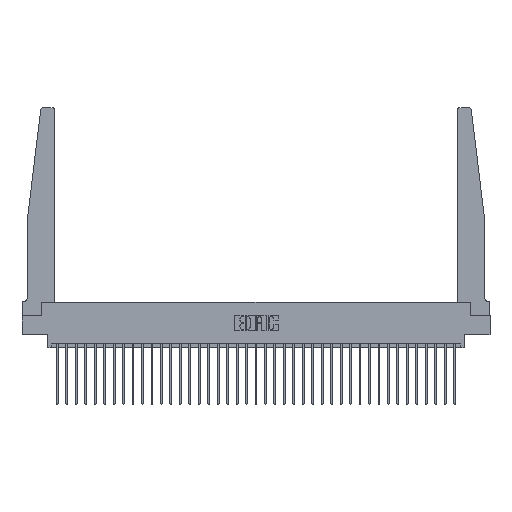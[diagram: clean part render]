
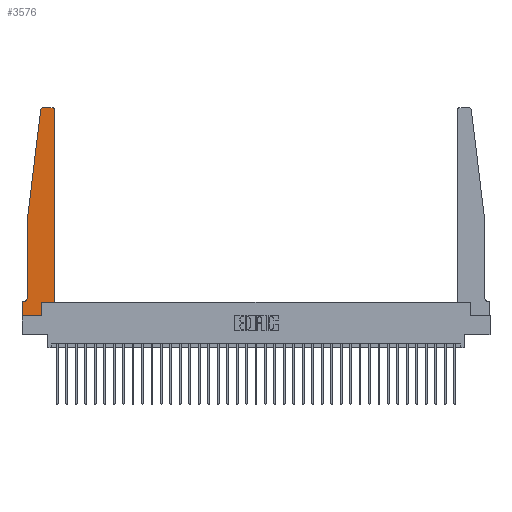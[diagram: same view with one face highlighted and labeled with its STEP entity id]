
A CAD part, top view. The second image highlights one B-rep face of the part: STEP entity #3576.
In plain terms, the highlighted planar face has unit normal (0, 0, 1).
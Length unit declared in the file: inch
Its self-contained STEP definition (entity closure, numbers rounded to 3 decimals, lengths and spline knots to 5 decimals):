
#4 = EDGE_CURVE ( 'NONE', #29340, #1644, #8275, .T. ) ;
#60 = CARTESIAN_POINT ( 'NONE',  ( 0.25, 2.75, 0.37 ) ) ;
#529 = VECTOR ( 'NONE', #12540, 39.37008 ) ;
#1047 = LINE ( 'NONE', #10996, #31137 ) ;
#1213 = EDGE_CURVE ( 'NONE', #19948, #30841, #32420, .T. ) ;
#1644 = VERTEX_POINT ( 'NONE', #14336 ) ;
#1823 = EDGE_CURVE ( 'NONE', #9716, #26521, #4570, .T. ) ;
#2283 = CARTESIAN_POINT ( 'NONE',  ( 0.425, 0.18, 0.37 ) ) ;
#2417 = EDGE_CURVE ( 'NONE', #14620, #32169, #27530, .T. ) ;
#2706 = LINE ( 'NONE', #31179, #25976 ) ;
#2826 = VERTEX_POINT ( 'NONE', #11321 ) ;
#3506 = CARTESIAN_POINT ( 'NONE',  ( 0.425, 0.18, 0.37 ) ) ;
#3576 = ADVANCED_FACE ( 'NONE', ( #8250 ), #26257, .T. ) ;
#3982 = CARTESIAN_POINT ( 'NONE',  ( 0., 0.1875, 0.37 ) ) ;
#4303 = CARTESIAN_POINT ( 'NONE',  ( 0.425, 0.18, 0.37 ) ) ;
#4419 = AXIS2_PLACEMENT_3D ( 'NONE', #22112, #9162, #19418 ) ;
#4570 = CIRCLE ( 'NONE', #27695, 0.03 ) ;
#5114 = VERTEX_POINT ( 'NONE', #31944 ) ;
#5246 = VECTOR ( 'NONE', #18828, 39.37008 ) ;
#5378 = CARTESIAN_POINT ( 'NONE',  ( 0.27653, 2.75, 0.37 ) ) ;
#5499 = VECTOR ( 'NONE', #24867, 39.37008 ) ;
#6516 = EDGE_CURVE ( 'NONE', #22549, #29228, #6541, .T. ) ;
#6541 = LINE ( 'NONE', #3506, #5246 ) ;
#7012 = EDGE_CURVE ( 'NONE', #2826, #9716, #23143, .T. ) ;
#8112 = DIRECTION ( 'NONE',  ( 0., -1., 0. ) ) ;
#8250 = FACE_OUTER_BOUND ( 'NONE', #9260, .T. ) ;
#8275 = LINE ( 'NONE', #22957, #25013 ) ;
#8446 = AXIS2_PLACEMENT_3D ( 'NONE', #16323, #12546, #13643 ) ;
#9051 = ORIENTED_EDGE ( 'NONE', *, *, #1823, .T. ) ;
#9140 = ORIENTED_EDGE ( 'NONE', *, *, #16018, .T. ) ;
#9162 = DIRECTION ( 'NONE',  ( 0., 0., 1. ) ) ;
#9260 = EDGE_LOOP ( 'NONE', ( #15042, #9051, #15859, #21249, #15495, #17906, #9140, #28413, #26639, #24978, #23606, #23764 ) ) ;
#9641 = VECTOR ( 'NONE', #27364, 39.37008 ) ;
#9716 = VERTEX_POINT ( 'NONE', #5378 ) ;
#10996 = CARTESIAN_POINT ( 'NONE',  ( 0.065, 1.25, 0.37 ) ) ;
#11321 = CARTESIAN_POINT ( 'NONE',  ( 0.395, 2.75, 0.37 ) ) ;
#12503 = CARTESIAN_POINT ( 'NONE',  ( 0.015, 0.1875, 0.37 ) ) ;
#12540 = DIRECTION ( 'NONE',  ( -1., 0., 0. ) ) ;
#12546 = DIRECTION ( 'NONE',  ( 0., 0., -1. ) ) ;
#12800 = EDGE_CURVE ( 'NONE', #29228, #2826, #18846, .T. ) ;
#13643 = DIRECTION ( 'NONE',  ( -1., 0., 0. ) ) ;
#14336 = CARTESIAN_POINT ( 'NONE',  ( 0.065, 0.2375, 0.37 ) ) ;
#14386 = VECTOR ( 'NONE', #24831, 39.37008 ) ;
#14620 = VERTEX_POINT ( 'NONE', #27475 ) ;
#14715 = CARTESIAN_POINT ( 'NONE',  ( 0.065, 0.1875, 0.37 ) ) ;
#14753 = EDGE_CURVE ( 'NONE', #5114, #14620, #2706, .T. ) ;
#14913 = CARTESIAN_POINT ( 'NONE',  ( 0.425, 2.72, 0.37 ) ) ;
#15042 = ORIENTED_EDGE ( 'NONE', *, *, #7012, .T. ) ;
#15495 = ORIENTED_EDGE ( 'NONE', *, *, #26215, .T. ) ;
#15660 = CARTESIAN_POINT ( 'NONE',  ( 0., 0., 0.37 ) ) ;
#15810 = DIRECTION ( 'NONE',  ( 0., 0., 1. ) ) ;
#15841 = CARTESIAN_POINT ( 'NONE',  ( 0.27653, 2.72, 0.37 ) ) ;
#15859 = ORIENTED_EDGE ( 'NONE', *, *, #27812, .T. ) ;
#16018 = EDGE_CURVE ( 'NONE', #30841, #5114, #28796, .T. ) ;
#16323 = CARTESIAN_POINT ( 'NONE',  ( 0.015, 0.2375, 0.37 ) ) ;
#17433 = LINE ( 'NONE', #4303, #5499 ) ;
#17906 = ORIENTED_EDGE ( 'NONE', *, *, #1213, .T. ) ;
#18192 = EDGE_CURVE ( 'NONE', #32169, #22549, #17433, .T. ) ;
#18496 = CARTESIAN_POINT ( 'NONE',  ( 0., 0.1875, 0.37 ) ) ;
#18731 = DIRECTION ( 'NONE',  ( -0.122, -0.992, 0. ) ) ;
#18828 = DIRECTION ( 'NONE',  ( 0., 1., 0. ) ) ;
#18846 = CIRCLE ( 'NONE', #4419, 0.03 ) ;
#19418 = DIRECTION ( 'NONE',  ( 1., 0., 0. ) ) ;
#19948 = VERTEX_POINT ( 'NONE', #12503 ) ;
#21249 = ORIENTED_EDGE ( 'NONE', *, *, #4, .T. ) ;
#21684 = DIRECTION ( 'NONE',  ( 1., 0., 0. ) ) ;
#22112 = CARTESIAN_POINT ( 'NONE',  ( 0.395, 2.72, 0.37 ) ) ;
#22549 = VERTEX_POINT ( 'NONE', #2283 ) ;
#22957 = CARTESIAN_POINT ( 'NONE',  ( 0.065, 1.25, 0.37 ) ) ;
#23143 = LINE ( 'NONE', #60, #14386 ) ;
#23606 = ORIENTED_EDGE ( 'NONE', *, *, #6516, .T. ) ;
#23764 = ORIENTED_EDGE ( 'NONE', *, *, #12800, .T. ) ;
#24831 = DIRECTION ( 'NONE',  ( -1., 0., 0. ) ) ;
#24867 = DIRECTION ( 'NONE',  ( 1., 0., 0. ) ) ;
#24978 = ORIENTED_EDGE ( 'NONE', *, *, #18192, .T. ) ;
#25013 = VECTOR ( 'NONE', #8112, 39.37008 ) ;
#25096 = CARTESIAN_POINT ( 'NONE',  ( 0.24675, 2.72367, 0.37 ) ) ;
#25390 = CARTESIAN_POINT ( 'NONE',  ( 0.2605, 0.18, 0.37 ) ) ;
#25957 = DIRECTION ( 'NONE',  ( 1., 0., 0. ) ) ;
#25976 = VECTOR ( 'NONE', #25957, 39.37008 ) ;
#26166 = AXIS2_PLACEMENT_3D ( 'NONE', #18496, #15810, #21684 ) ;
#26215 = EDGE_CURVE ( 'NONE', #1644, #19948, #26737, .T. ) ;
#26257 = PLANE ( 'NONE',  #26166 ) ;
#26521 = VERTEX_POINT ( 'NONE', #25096 ) ;
#26639 = ORIENTED_EDGE ( 'NONE', *, *, #2417, .T. ) ;
#26737 = CIRCLE ( 'NONE', #8446, 0.05 ) ;
#27364 = DIRECTION ( 'NONE',  ( 0., 1., 0. ) ) ;
#27475 = CARTESIAN_POINT ( 'NONE',  ( 0.2605, 0., 0.37 ) ) ;
#27530 = LINE ( 'NONE', #30403, #9641 ) ;
#27695 = AXIS2_PLACEMENT_3D ( 'NONE', #15841, #33060, #30860 ) ;
#27812 = EDGE_CURVE ( 'NONE', #26521, #29340, #1047, .T. ) ;
#28141 = DIRECTION ( 'NONE',  ( 0., -1., 0. ) ) ;
#28413 = ORIENTED_EDGE ( 'NONE', *, *, #14753, .T. ) ;
#28796 = LINE ( 'NONE', #15660, #32457 ) ;
#29228 = VERTEX_POINT ( 'NONE', #14913 ) ;
#29340 = VERTEX_POINT ( 'NONE', #31416 ) ;
#30403 = CARTESIAN_POINT ( 'NONE',  ( 0.2605, 0.18, 0.37 ) ) ;
#30841 = VERTEX_POINT ( 'NONE', #3982 ) ;
#30860 = DIRECTION ( 'NONE',  ( 1., 0., 0. ) ) ;
#31137 = VECTOR ( 'NONE', #18731, 39.37008 ) ;
#31179 = CARTESIAN_POINT ( 'NONE',  ( 0., 0., 0.37 ) ) ;
#31416 = CARTESIAN_POINT ( 'NONE',  ( 0.065, 1.25, 0.37 ) ) ;
#31944 = CARTESIAN_POINT ( 'NONE',  ( 0., 0., 0.37 ) ) ;
#32169 = VERTEX_POINT ( 'NONE', #25390 ) ;
#32420 = LINE ( 'NONE', #14715, #529 ) ;
#32457 = VECTOR ( 'NONE', #28141, 39.37008 ) ;
#33060 = DIRECTION ( 'NONE',  ( 0., 0., 1. ) ) ;
